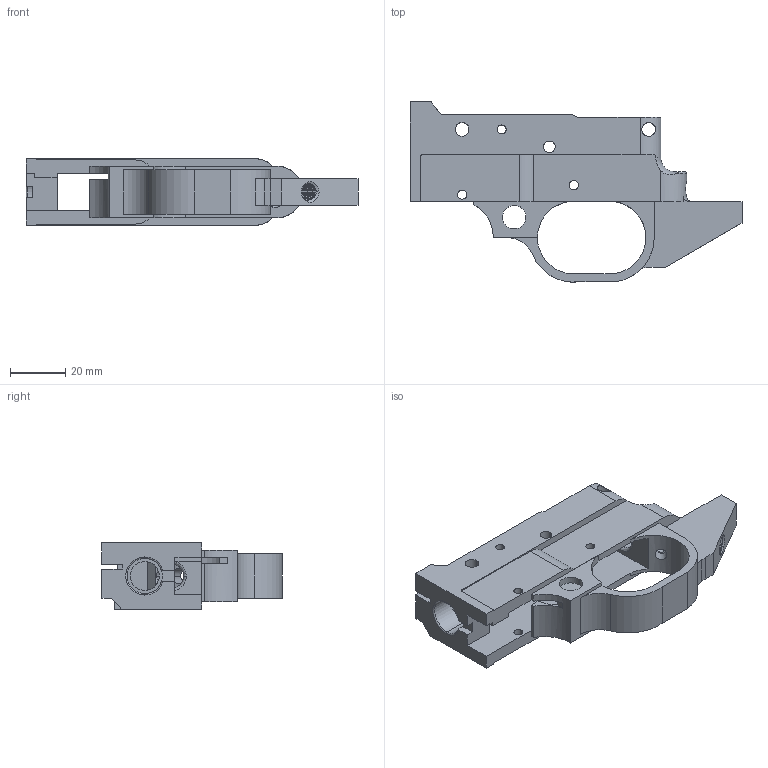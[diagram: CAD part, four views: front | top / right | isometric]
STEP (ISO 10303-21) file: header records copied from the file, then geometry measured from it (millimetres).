
FILE_DESCRIPTION (( 'STEP AP214' ), '1' );
FILE_NAME ('10-22 trigger pistol.STEP', '2015-05-08T20:11:21', ( 'WarFairy' ), ( '' ), 'SwSTEP 2.0', 'SolidWorks 2015', '' );
FILE_SCHEMA (( 'AUTOMOTIVE_DESIGN' ));
Length unit declared in the file: millimetre
Products named in the file (1): 10-22 trigger pistol
Bounding box: 120.06 x 65.17 x 24 mm (x, y, z)
Volume: 41805.9 mm3; surface area: 23450.6 mm2
Topology: 1 solids, 1 shells, 175 faces, 523 edges, 342 vertices
Faces by surface type: cylinder 83, plane 75, torus 10, bspline 5, cone 2
Entity records: 8477 total; most frequent: CARTESIAN_POINT 3794, ORIENTED_EDGE 1046, DIRECTION 917, EDGE_CURVE 523, VERTEX_POINT 342, AXIS2_PLACEMENT_3D 316, VECTOR 285, LINE 285
